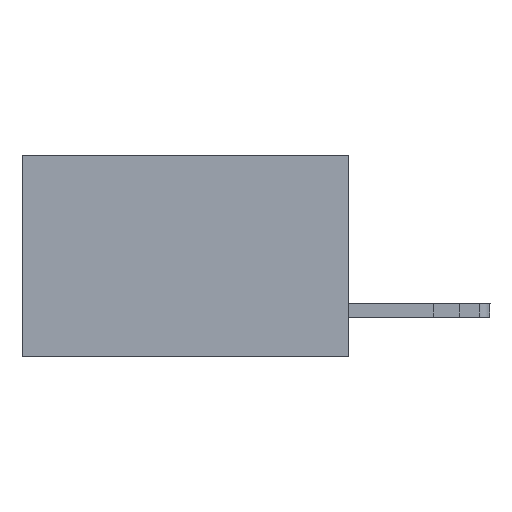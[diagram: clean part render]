
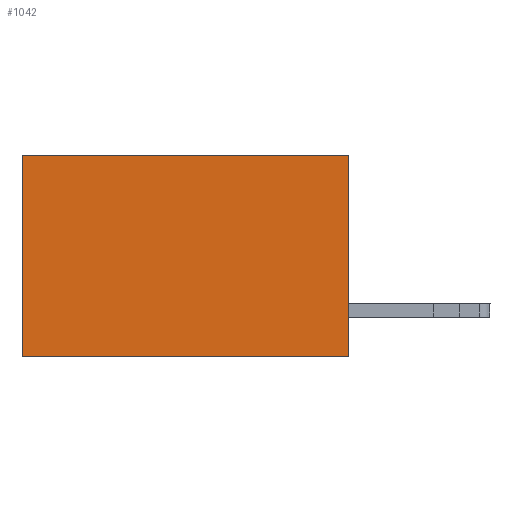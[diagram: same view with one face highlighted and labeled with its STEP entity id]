
A CAD part, left-side view. The second image highlights one B-rep face of the part: STEP entity #1042.
In plain terms, the highlighted planar face has unit normal (-1, 0, 0).
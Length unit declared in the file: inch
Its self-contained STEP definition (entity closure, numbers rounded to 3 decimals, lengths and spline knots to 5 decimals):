
#564 = EDGE_CURVE ( 'NONE', #11276, #7507, #12012, .T. ) ;
#945 = AXIS2_PLACEMENT_3D ( 'NONE', #4106, #2669, #8694 ) ;
#1042 = ADVANCED_FACE ( 'NONE', ( #12573 ), #2685, .F. ) ;
#1101 = LINE ( 'NONE', #3341, #12979 ) ;
#1616 = ORIENTED_EDGE ( 'NONE', *, *, #4119, .T. ) ;
#2543 = ORIENTED_EDGE ( 'NONE', *, *, #10899, .F. ) ;
#2669 = DIRECTION ( 'NONE',  ( 1., 0., 0. ) ) ;
#2685 = PLANE ( 'NONE',  #945 ) ;
#2703 = VERTEX_POINT ( 'NONE', #8379 ) ;
#3286 = ORIENTED_EDGE ( 'NONE', *, *, #10399, .F. ) ;
#3341 = CARTESIAN_POINT ( 'NONE',  ( 0.2615, 0.6, -0.37 ) ) ;
#3679 = VECTOR ( 'NONE', #9470, 39.37008 ) ;
#4106 = CARTESIAN_POINT ( 'NONE',  ( 0.2615, 0., -0.37 ) ) ;
#4119 = EDGE_CURVE ( 'NONE', #7507, #2703, #1101, .T. ) ;
#4272 = CARTESIAN_POINT ( 'NONE',  ( 0.2615, 0.6, 0. ) ) ;
#4954 = DIRECTION ( 'NONE',  ( 0., 1., 0. ) ) ;
#6381 = VECTOR ( 'NONE', #4954, 39.37008 ) ;
#7432 = VERTEX_POINT ( 'NONE', #7683 ) ;
#7507 = VERTEX_POINT ( 'NONE', #4272 ) ;
#7633 = LINE ( 'NONE', #14732, #3679 ) ;
#7683 = CARTESIAN_POINT ( 'NONE',  ( 0.2615, 0., -0.37 ) ) ;
#8041 = EDGE_LOOP ( 'NONE', ( #1616, #3286, #2543, #13585 ) ) ;
#8379 = CARTESIAN_POINT ( 'NONE',  ( 0.2615, 0.6, -0.37 ) ) ;
#8694 = DIRECTION ( 'NONE',  ( 0., 0., -1. ) ) ;
#8773 = VECTOR ( 'NONE', #12064, 39.37008 ) ;
#8830 = CARTESIAN_POINT ( 'NONE',  ( 0.2615, 0., 0. ) ) ;
#8972 = LINE ( 'NONE', #11697, #6381 ) ;
#9470 = DIRECTION ( 'NONE',  ( 0., 0., -1. ) ) ;
#10329 = CARTESIAN_POINT ( 'NONE',  ( 0.2615, 0., 0. ) ) ;
#10399 = EDGE_CURVE ( 'NONE', #7432, #2703, #8972, .T. ) ;
#10899 = EDGE_CURVE ( 'NONE', #11276, #7432, #7633, .T. ) ;
#11276 = VERTEX_POINT ( 'NONE', #8830 ) ;
#11697 = CARTESIAN_POINT ( 'NONE',  ( 0.2615, 0., -0.37 ) ) ;
#11937 = DIRECTION ( 'NONE',  ( 0., 0., -1. ) ) ;
#12012 = LINE ( 'NONE', #10329, #8773 ) ;
#12064 = DIRECTION ( 'NONE',  ( 0., 1., 0. ) ) ;
#12573 = FACE_OUTER_BOUND ( 'NONE', #8041, .T. ) ;
#12979 = VECTOR ( 'NONE', #11937, 39.37008 ) ;
#13585 = ORIENTED_EDGE ( 'NONE', *, *, #564, .T. ) ;
#14732 = CARTESIAN_POINT ( 'NONE',  ( 0.2615, 0., -0.37 ) ) ;
